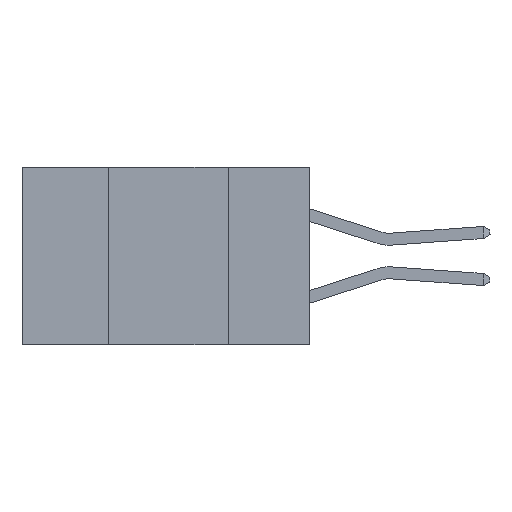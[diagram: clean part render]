
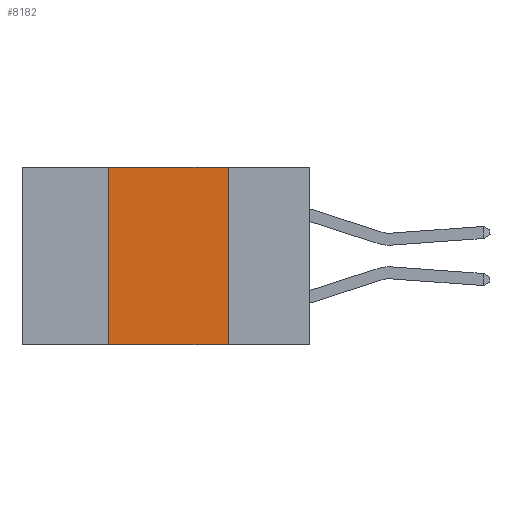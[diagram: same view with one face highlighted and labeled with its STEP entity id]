
A CAD part, left-side view. The second image highlights one B-rep face of the part: STEP entity #8182.
In plain terms, the highlighted planar face has unit normal (-1, 0, 0).
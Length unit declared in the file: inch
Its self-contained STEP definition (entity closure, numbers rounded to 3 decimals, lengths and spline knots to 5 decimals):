
#218 = EDGE_CURVE ( 'NONE', #2085, #362, #3035, .T. ) ;
#362 = VERTEX_POINT ( 'NONE', #11782 ) ;
#2085 = VERTEX_POINT ( 'NONE', #15462 ) ;
#2656 = DIRECTION ( 'NONE',  ( 0., -1., 0. ) ) ;
#2678 = ORIENTED_EDGE ( 'NONE', *, *, #5352, .F. ) ;
#3035 = LINE ( 'NONE', #24775, #3315 ) ;
#3315 = VECTOR ( 'NONE', #2656, 39.37008 ) ;
#3350 = VECTOR ( 'NONE', #18808, 39.37008 ) ;
#3383 = VECTOR ( 'NONE', #21125, 39.37008 ) ;
#5352 = EDGE_CURVE ( 'NONE', #25061, #12188, #6634, .T. ) ;
#5592 = EDGE_CURVE ( 'NONE', #12188, #362, #17465, .T. ) ;
#6504 = CARTESIAN_POINT ( 'NONE',  ( 0., 0.6, 0. ) ) ;
#6634 = LINE ( 'NONE', #6504, #3350 ) ;
#7015 = CARTESIAN_POINT ( 'NONE',  ( 0., 0.17, -0.37 ) ) ;
#7654 = AXIS2_PLACEMENT_3D ( 'NONE', #13411, #17213, #17737 ) ;
#8182 = ADVANCED_FACE ( 'NONE', ( #23362 ), #13280, .F. ) ;
#9046 = CARTESIAN_POINT ( 'NONE',  ( 0., 0.17, 0. ) ) ;
#9167 = CARTESIAN_POINT ( 'NONE',  ( 0., 0.42, -0.37 ) ) ;
#9541 = EDGE_LOOP ( 'NONE', ( #18213, #2678, #10869, #25300 ) ) ;
#10869 = ORIENTED_EDGE ( 'NONE', *, *, #17135, .F. ) ;
#11782 = CARTESIAN_POINT ( 'NONE',  ( 0., 0.17, -0.37 ) ) ;
#12188 = VERTEX_POINT ( 'NONE', #9046 ) ;
#13280 = PLANE ( 'NONE',  #7654 ) ;
#13411 = CARTESIAN_POINT ( 'NONE',  ( 0., 0.6, 0. ) ) ;
#15462 = CARTESIAN_POINT ( 'NONE',  ( 0., 0.42, -0.37 ) ) ;
#17135 = EDGE_CURVE ( 'NONE', #2085, #25061, #19113, .T. ) ;
#17213 = DIRECTION ( 'NONE',  ( 1., 0., 0. ) ) ;
#17465 = LINE ( 'NONE', #7015, #3383 ) ;
#17737 = DIRECTION ( 'NONE',  ( 0., 0., -1. ) ) ;
#18213 = ORIENTED_EDGE ( 'NONE', *, *, #5592, .F. ) ;
#18808 = DIRECTION ( 'NONE',  ( 0., -1., 0. ) ) ;
#19113 = LINE ( 'NONE', #9167, #22518 ) ;
#21125 = DIRECTION ( 'NONE',  ( 0., 0., -1. ) ) ;
#22518 = VECTOR ( 'NONE', #24741, 39.37008 ) ;
#23362 = FACE_OUTER_BOUND ( 'NONE', #9541, .T. ) ;
#23902 = CARTESIAN_POINT ( 'NONE',  ( 0., 0.42, 0. ) ) ;
#24741 = DIRECTION ( 'NONE',  ( 0., 0., 1. ) ) ;
#24775 = CARTESIAN_POINT ( 'NONE',  ( 0., 0.6, -0.37 ) ) ;
#25061 = VERTEX_POINT ( 'NONE', #23902 ) ;
#25300 = ORIENTED_EDGE ( 'NONE', *, *, #218, .T. ) ;
